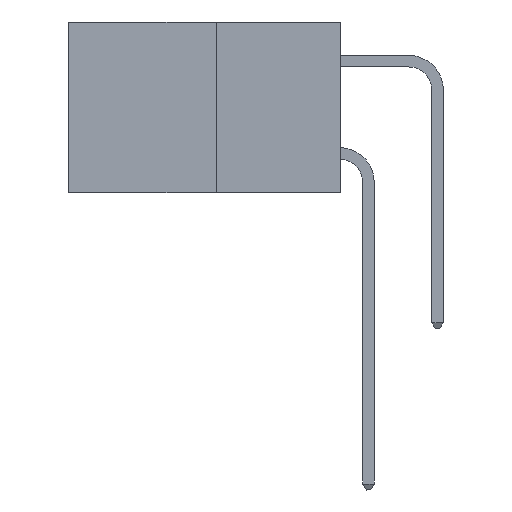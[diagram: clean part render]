
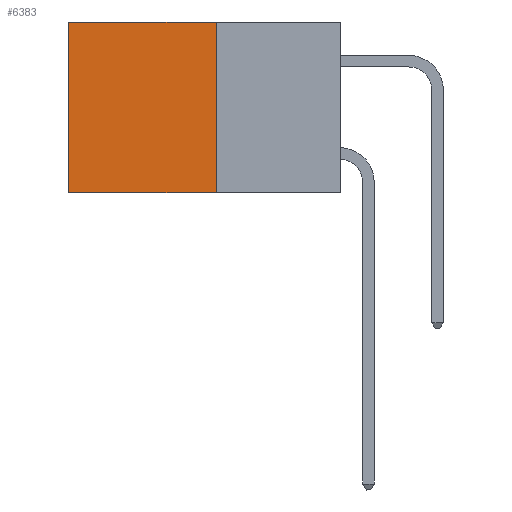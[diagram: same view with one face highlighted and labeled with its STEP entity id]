
A CAD part, left-side view. The second image highlights one B-rep face of the part: STEP entity #6383.
In plain terms, the highlighted planar face has unit normal (-1, 0, 0).
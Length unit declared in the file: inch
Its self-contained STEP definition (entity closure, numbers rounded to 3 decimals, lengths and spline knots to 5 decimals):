
#283 = VECTOR ( 'NONE', #7418, 39.37008 ) ;
#1602 = DIRECTION ( 'NONE',  ( 0., 1., 0. ) ) ;
#1645 = CARTESIAN_POINT ( 'NONE',  ( 0.277, 0.27, 0. ) ) ;
#1853 = VERTEX_POINT ( 'NONE', #5184 ) ;
#2580 = LINE ( 'NONE', #11567, #14540 ) ;
#3772 = CARTESIAN_POINT ( 'NONE',  ( 0.277, 0.59, 0. ) ) ;
#4086 = EDGE_CURVE ( 'NONE', #9883, #5534, #13661, .T. ) ;
#4387 = VECTOR ( 'NONE', #7401, 39.37008 ) ;
#4931 = EDGE_LOOP ( 'NONE', ( #8835, #6122, #9926, #7574 ) ) ;
#5164 = AXIS2_PLACEMENT_3D ( 'NONE', #12049, #11428, #11415 ) ;
#5184 = CARTESIAN_POINT ( 'NONE',  ( 0.277, 0.27, 0. ) ) ;
#5534 = VERTEX_POINT ( 'NONE', #7771 ) ;
#6122 = ORIENTED_EDGE ( 'NONE', *, *, #4086, .F. ) ;
#6383 = ADVANCED_FACE ( 'NONE', ( #14276 ), #12066, .F. ) ;
#7266 = CARTESIAN_POINT ( 'NONE',  ( 0.277, 0.59, -0.37 ) ) ;
#7401 = DIRECTION ( 'NONE',  ( 0., 1., 0. ) ) ;
#7418 = DIRECTION ( 'NONE',  ( 0., 0., -1. ) ) ;
#7574 = ORIENTED_EDGE ( 'NONE', *, *, #8117, .T. ) ;
#7771 = CARTESIAN_POINT ( 'NONE',  ( 0.277, 0.59, -0.37 ) ) ;
#8117 = EDGE_CURVE ( 'NONE', #1853, #11907, #10142, .T. ) ;
#8653 = CARTESIAN_POINT ( 'NONE',  ( 0.277, 0.27, -0.37 ) ) ;
#8800 = EDGE_CURVE ( 'NONE', #11907, #5534, #9206, .T. ) ;
#8835 = ORIENTED_EDGE ( 'NONE', *, *, #8800, .T. ) ;
#9206 = LINE ( 'NONE', #7266, #283 ) ;
#9722 = EDGE_CURVE ( 'NONE', #1853, #9883, #2580, .T. ) ;
#9883 = VERTEX_POINT ( 'NONE', #10395 ) ;
#9926 = ORIENTED_EDGE ( 'NONE', *, *, #9722, .F. ) ;
#10142 = LINE ( 'NONE', #1645, #12486 ) ;
#10395 = CARTESIAN_POINT ( 'NONE',  ( 0.277, 0.27, -0.37 ) ) ;
#11415 = DIRECTION ( 'NONE',  ( 0., 0., -1. ) ) ;
#11428 = DIRECTION ( 'NONE',  ( 1., 0., 0. ) ) ;
#11483 = DIRECTION ( 'NONE',  ( 0., 0., -1. ) ) ;
#11567 = CARTESIAN_POINT ( 'NONE',  ( 0.277, 0.27, -0.37 ) ) ;
#11907 = VERTEX_POINT ( 'NONE', #3772 ) ;
#12049 = CARTESIAN_POINT ( 'NONE',  ( 0.277, 0.27, -0.37 ) ) ;
#12066 = PLANE ( 'NONE',  #5164 ) ;
#12486 = VECTOR ( 'NONE', #1602, 39.37008 ) ;
#13661 = LINE ( 'NONE', #8653, #4387 ) ;
#14276 = FACE_OUTER_BOUND ( 'NONE', #4931, .T. ) ;
#14540 = VECTOR ( 'NONE', #11483, 39.37008 ) ;
